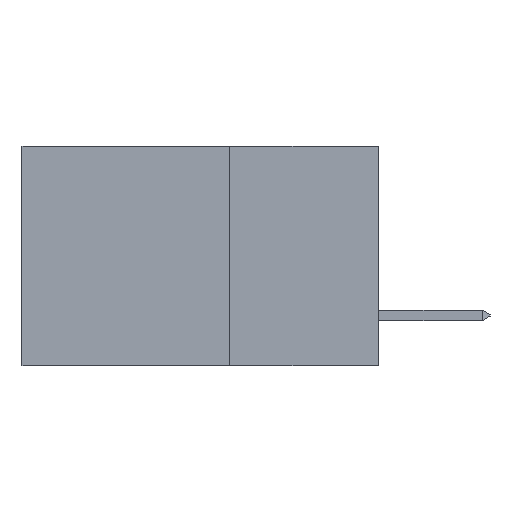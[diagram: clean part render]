
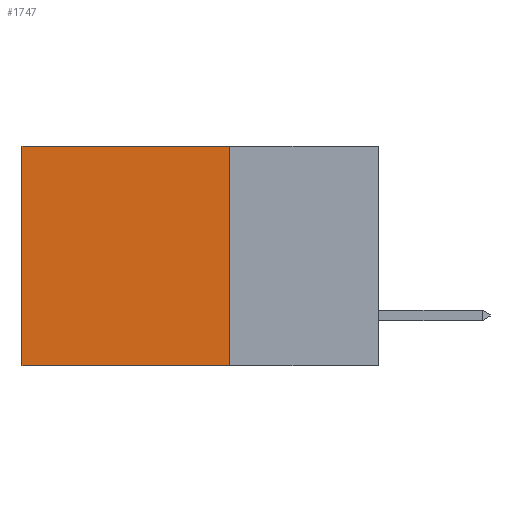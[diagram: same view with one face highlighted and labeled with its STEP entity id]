
A CAD part, left-side view. The second image highlights one B-rep face of the part: STEP entity #1747.
In plain terms, the highlighted planar face has unit normal (-1, 0, 0).
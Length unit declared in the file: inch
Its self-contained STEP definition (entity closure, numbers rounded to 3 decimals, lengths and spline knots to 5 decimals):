
#238 = LINE ( 'NONE', #10056, #3350 ) ;
#909 = LINE ( 'NONE', #13728, #4417 ) ;
#935 = VECTOR ( 'NONE', #13777, 39.37008 ) ;
#1205 = VERTEX_POINT ( 'NONE', #6980 ) ;
#1460 = DIRECTION ( 'NONE',  ( 1., 0., 0. ) ) ;
#1747 = ADVANCED_FACE ( 'NONE', ( #10431 ), #15347, .F. ) ;
#1792 = VERTEX_POINT ( 'NONE', #11527 ) ;
#1828 = VERTEX_POINT ( 'NONE', #3658 ) ;
#2169 = ORIENTED_EDGE ( 'NONE', *, *, #16260, .F. ) ;
#2927 = CARTESIAN_POINT ( 'NONE',  ( 0.2615, 0.25, -0.37 ) ) ;
#3350 = VECTOR ( 'NONE', #4879, 39.37008 ) ;
#3658 = CARTESIAN_POINT ( 'NONE',  ( 0.2615, 0.25, 0. ) ) ;
#4030 = ORIENTED_EDGE ( 'NONE', *, *, #13098, .F. ) ;
#4417 = VECTOR ( 'NONE', #14075, 39.37008 ) ;
#4437 = LINE ( 'NONE', #12516, #935 ) ;
#4843 = VERTEX_POINT ( 'NONE', #2927 ) ;
#4879 = DIRECTION ( 'NONE',  ( 0., 1., 0. ) ) ;
#6200 = AXIS2_PLACEMENT_3D ( 'NONE', #9320, #1460, #16646 ) ;
#6980 = CARTESIAN_POINT ( 'NONE',  ( 0.2615, 0.6, 0. ) ) ;
#7371 = LINE ( 'NONE', #12457, #13766 ) ;
#9320 = CARTESIAN_POINT ( 'NONE',  ( 0.2615, 0.25, -0.37 ) ) ;
#9789 = EDGE_CURVE ( 'NONE', #1205, #1792, #909, .T. ) ;
#10056 = CARTESIAN_POINT ( 'NONE',  ( 0.2615, 0.25, 0. ) ) ;
#10431 = FACE_OUTER_BOUND ( 'NONE', #12579, .T. ) ;
#11356 = EDGE_CURVE ( 'NONE', #1828, #1205, #238, .T. ) ;
#11527 = CARTESIAN_POINT ( 'NONE',  ( 0.2615, 0.6, -0.37 ) ) ;
#12457 = CARTESIAN_POINT ( 'NONE',  ( 0.2615, 0.25, -0.37 ) ) ;
#12516 = CARTESIAN_POINT ( 'NONE',  ( 0.2615, 0.25, -0.37 ) ) ;
#12579 = EDGE_LOOP ( 'NONE', ( #15882, #2169, #4030, #13136 ) ) ;
#13098 = EDGE_CURVE ( 'NONE', #1828, #4843, #7371, .T. ) ;
#13136 = ORIENTED_EDGE ( 'NONE', *, *, #11356, .T. ) ;
#13724 = DIRECTION ( 'NONE',  ( 0., 0., -1. ) ) ;
#13728 = CARTESIAN_POINT ( 'NONE',  ( 0.2615, 0.6, -0.37 ) ) ;
#13766 = VECTOR ( 'NONE', #13724, 39.37008 ) ;
#13777 = DIRECTION ( 'NONE',  ( 0., 1., 0. ) ) ;
#14075 = DIRECTION ( 'NONE',  ( 0., 0., -1. ) ) ;
#15347 = PLANE ( 'NONE',  #6200 ) ;
#15882 = ORIENTED_EDGE ( 'NONE', *, *, #9789, .T. ) ;
#16260 = EDGE_CURVE ( 'NONE', #4843, #1792, #4437, .T. ) ;
#16646 = DIRECTION ( 'NONE',  ( 0., 0., -1. ) ) ;
